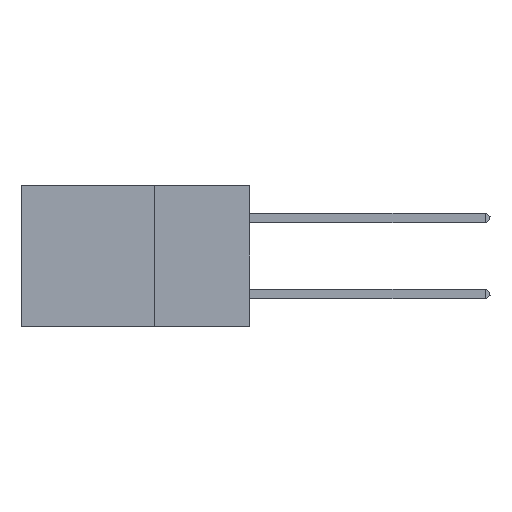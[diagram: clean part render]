
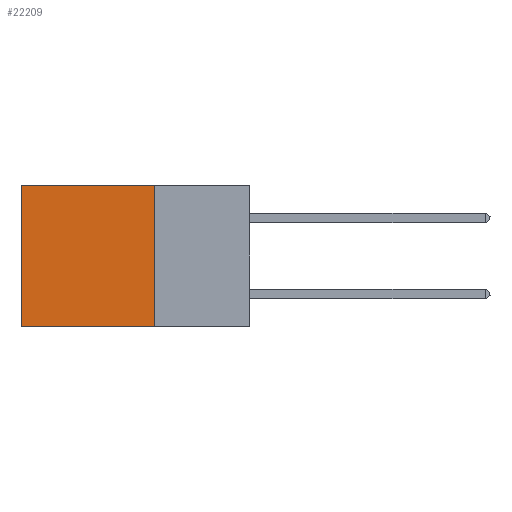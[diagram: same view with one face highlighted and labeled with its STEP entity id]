
A CAD part, left-side view. The second image highlights one B-rep face of the part: STEP entity #22209.
In plain terms, the highlighted planar face has unit normal (-1, 0, 0).
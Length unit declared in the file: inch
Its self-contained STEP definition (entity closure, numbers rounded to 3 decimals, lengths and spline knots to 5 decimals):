
#2427 = AXIS2_PLACEMENT_3D ( 'NONE', #3299, #28502, #6972 ) ;
#2867 = CARTESIAN_POINT ( 'NONE',  ( 0.2875, 0.25, 0. ) ) ;
#3258 = VERTEX_POINT ( 'NONE', #20744 ) ;
#3299 = CARTESIAN_POINT ( 'NONE',  ( 0.2875, 0.25, 0. ) ) ;
#4980 = VERTEX_POINT ( 'NONE', #2867 ) ;
#6972 = DIRECTION ( 'NONE',  ( 0., 0., -1. ) ) ;
#9167 = CARTESIAN_POINT ( 'NONE',  ( 0.2875, 0.25, 0. ) ) ;
#11440 = CARTESIAN_POINT ( 'NONE',  ( 0.2875, 0.25, -0.37 ) ) ;
#12621 = EDGE_CURVE ( 'NONE', #4980, #33869, #35333, .T. ) ;
#13254 = ORIENTED_EDGE ( 'NONE', *, *, #18142, .T. ) ;
#15269 = EDGE_CURVE ( 'NONE', #33869, #3258, #36745, .T. ) ;
#18064 = LINE ( 'NONE', #20883, #38617 ) ;
#18142 = EDGE_CURVE ( 'NONE', #39140, #3258, #44118, .T. ) ;
#20744 = CARTESIAN_POINT ( 'NONE',  ( 0.2875, 0.6, -0.37 ) ) ;
#20883 = CARTESIAN_POINT ( 'NONE',  ( 0.2875, 0.25, 0. ) ) ;
#21907 = VECTOR ( 'NONE', #22332, 39.37008 ) ;
#22209 = ADVANCED_FACE ( 'NONE', ( #32256 ), #25125, .F. ) ;
#22332 = DIRECTION ( 'NONE',  ( 0., 1., 0. ) ) ;
#25000 = DIRECTION ( 'NONE',  ( 0., 1., 0. ) ) ;
#25125 = PLANE ( 'NONE',  #2427 ) ;
#25756 = ORIENTED_EDGE ( 'NONE', *, *, #46388, .T. ) ;
#27509 = DIRECTION ( 'NONE',  ( 0., 0., -1. ) ) ;
#28502 = DIRECTION ( 'NONE',  ( 1., 0., 0. ) ) ;
#32097 = VECTOR ( 'NONE', #32792, 39.37008 ) ;
#32256 = FACE_OUTER_BOUND ( 'NONE', #44057, .T. ) ;
#32671 = CARTESIAN_POINT ( 'NONE',  ( 0.2875, 0.6, 0. ) ) ;
#32792 = DIRECTION ( 'NONE',  ( 0., 0., -1. ) ) ;
#33869 = VERTEX_POINT ( 'NONE', #11440 ) ;
#35333 = LINE ( 'NONE', #9167, #41606 ) ;
#36745 = LINE ( 'NONE', #43612, #21907 ) ;
#38538 = ORIENTED_EDGE ( 'NONE', *, *, #15269, .F. ) ;
#38617 = VECTOR ( 'NONE', #25000, 39.37008 ) ;
#39140 = VERTEX_POINT ( 'NONE', #32671 ) ;
#39975 = ORIENTED_EDGE ( 'NONE', *, *, #12621, .F. ) ;
#41606 = VECTOR ( 'NONE', #27509, 39.37008 ) ;
#43612 = CARTESIAN_POINT ( 'NONE',  ( 0.2875, 0.25, -0.37 ) ) ;
#43823 = CARTESIAN_POINT ( 'NONE',  ( 0.2875, 0.6, 0. ) ) ;
#44057 = EDGE_LOOP ( 'NONE', ( #13254, #38538, #39975, #25756 ) ) ;
#44118 = LINE ( 'NONE', #43823, #32097 ) ;
#46388 = EDGE_CURVE ( 'NONE', #4980, #39140, #18064, .T. ) ;
